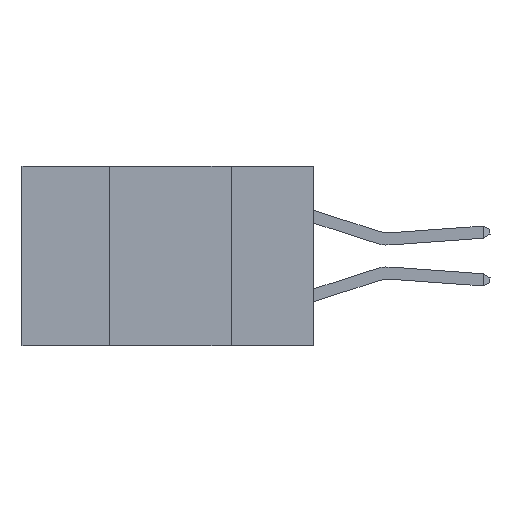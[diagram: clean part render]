
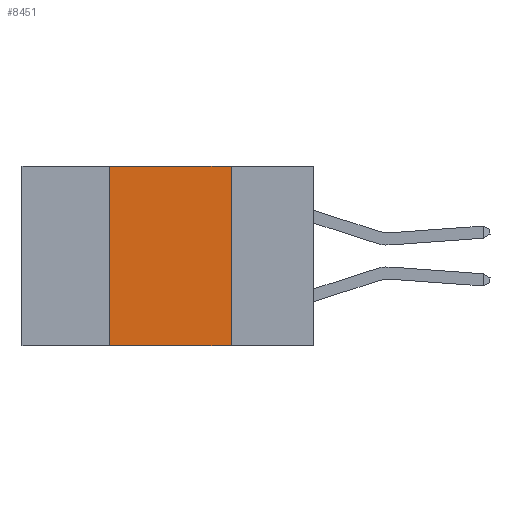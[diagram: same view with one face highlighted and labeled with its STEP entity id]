
A CAD part, left-side view. The second image highlights one B-rep face of the part: STEP entity #8451.
In plain terms, the highlighted planar face has unit normal (-1, 0, 0).
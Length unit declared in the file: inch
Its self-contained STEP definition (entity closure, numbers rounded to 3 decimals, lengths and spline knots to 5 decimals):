
#912 = ORIENTED_EDGE ( 'NONE', *, *, #27715, .F. ) ;
#1456 = CARTESIAN_POINT ( 'NONE',  ( 0., 0.6, 0. ) ) ;
#2092 = CARTESIAN_POINT ( 'NONE',  ( 0., 0.42, 0. ) ) ;
#3868 = VECTOR ( 'NONE', #4706, 39.37008 ) ;
#4493 = DIRECTION ( 'NONE',  ( 0., -1., 0. ) ) ;
#4706 = DIRECTION ( 'NONE',  ( 0., -1., 0. ) ) ;
#5828 = VERTEX_POINT ( 'NONE', #39660 ) ;
#5920 = VERTEX_POINT ( 'NONE', #15322 ) ;
#6294 = VECTOR ( 'NONE', #37727, 39.37008 ) ;
#7003 = ORIENTED_EDGE ( 'NONE', *, *, #19525, .F. ) ;
#8224 = VERTEX_POINT ( 'NONE', #13918 ) ;
#8307 = DIRECTION ( 'NONE',  ( 0., 0., -1. ) ) ;
#8451 = ADVANCED_FACE ( 'NONE', ( #24734 ), #40898, .F. ) ;
#10674 = LINE ( 'NONE', #21165, #3868 ) ;
#11236 = CARTESIAN_POINT ( 'NONE',  ( 0., 0.6, 0. ) ) ;
#13918 = CARTESIAN_POINT ( 'NONE',  ( 0., 0.42, -0.37 ) ) ;
#15322 = CARTESIAN_POINT ( 'NONE',  ( 0., 0.42, 0. ) ) ;
#16058 = VECTOR ( 'NONE', #4493, 39.37008 ) ;
#19525 = EDGE_CURVE ( 'NONE', #8224, #5920, #35532, .T. ) ;
#19851 = ORIENTED_EDGE ( 'NONE', *, *, #34143, .F. ) ;
#21165 = CARTESIAN_POINT ( 'NONE',  ( 0., 0.6, -0.37 ) ) ;
#21179 = EDGE_CURVE ( 'NONE', #8224, #27938, #10674, .T. ) ;
#24734 = FACE_OUTER_BOUND ( 'NONE', #35105, .T. ) ;
#26108 = VECTOR ( 'NONE', #29163, 39.37008 ) ;
#27715 = EDGE_CURVE ( 'NONE', #5828, #27938, #42000, .T. ) ;
#27938 = VERTEX_POINT ( 'NONE', #41377 ) ;
#29163 = DIRECTION ( 'NONE',  ( 0., 0., 1. ) ) ;
#30573 = CARTESIAN_POINT ( 'NONE',  ( 0., 0.17, 0. ) ) ;
#32125 = DIRECTION ( 'NONE',  ( 1., 0., 0. ) ) ;
#34143 = EDGE_CURVE ( 'NONE', #5920, #5828, #40222, .T. ) ;
#34862 = AXIS2_PLACEMENT_3D ( 'NONE', #1456, #32125, #8307 ) ;
#35105 = EDGE_LOOP ( 'NONE', ( #912, #19851, #7003, #37733 ) ) ;
#35532 = LINE ( 'NONE', #2092, #26108 ) ;
#37727 = DIRECTION ( 'NONE',  ( 0., 0., -1. ) ) ;
#37733 = ORIENTED_EDGE ( 'NONE', *, *, #21179, .T. ) ;
#39660 = CARTESIAN_POINT ( 'NONE',  ( 0., 0.17, 0. ) ) ;
#40222 = LINE ( 'NONE', #11236, #16058 ) ;
#40898 = PLANE ( 'NONE',  #34862 ) ;
#41377 = CARTESIAN_POINT ( 'NONE',  ( 0., 0.17, -0.37 ) ) ;
#42000 = LINE ( 'NONE', #30573, #6294 ) ;
